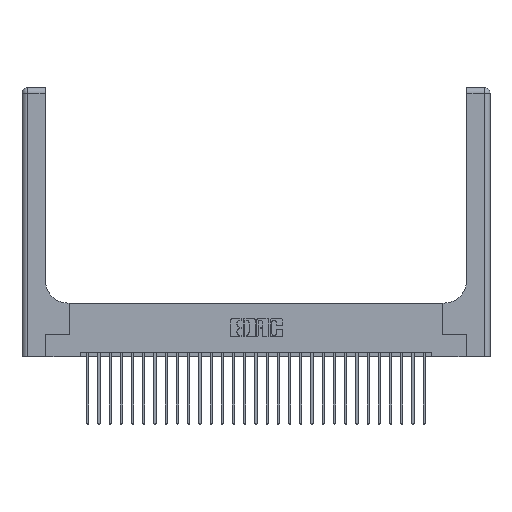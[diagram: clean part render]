
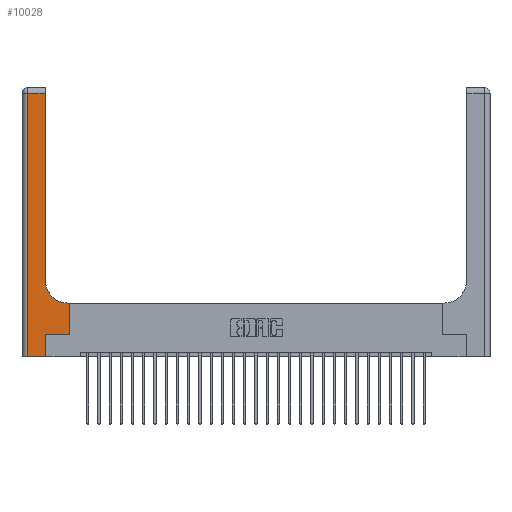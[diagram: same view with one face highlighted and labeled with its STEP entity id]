
A CAD part, top view. The second image highlights one B-rep face of the part: STEP entity #10028.
In plain terms, the highlighted planar face has unit normal (0, 0, 1).
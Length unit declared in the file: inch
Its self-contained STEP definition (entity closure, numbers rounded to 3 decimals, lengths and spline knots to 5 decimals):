
#576 = VERTEX_POINT ( 'NONE', #19433 ) ;
#1052 = CARTESIAN_POINT ( 'NONE',  ( 0.26, 2.94, 0.37 ) ) ;
#1129 = DIRECTION ( 'NONE',  ( 0., 1., 0. ) ) ;
#1941 = CARTESIAN_POINT ( 'NONE',  ( 0.06, 0., 0.37 ) ) ;
#2480 = LINE ( 'NONE', #8867, #11955 ) ;
#2795 = CARTESIAN_POINT ( 'NONE',  ( 0., 3., 0.37 ) ) ;
#3613 = AXIS2_PLACEMENT_3D ( 'NONE', #14170, #26631, #18584 ) ;
#3953 = CARTESIAN_POINT ( 'NONE',  ( 0.265, 0., 0.37 ) ) ;
#4069 = EDGE_CURVE ( 'NONE', #576, #4674, #22612, .T. ) ;
#4525 = ORIENTED_EDGE ( 'NONE', *, *, #26622, .T. ) ;
#4651 = LINE ( 'NONE', #19474, #24740 ) ;
#4674 = VERTEX_POINT ( 'NONE', #25059 ) ;
#4836 = VECTOR ( 'NONE', #20425, 39.37008 ) ;
#4862 = VECTOR ( 'NONE', #7663, 39.37008 ) ;
#5423 = EDGE_CURVE ( 'NONE', #5926, #25636, #27189, .T. ) ;
#5494 = VERTEX_POINT ( 'NONE', #24278 ) ;
#5569 = CARTESIAN_POINT ( 'NONE',  ( 0.51, 0.6, 0.37 ) ) ;
#5577 = VERTEX_POINT ( 'NONE', #5569 ) ;
#5926 = VERTEX_POINT ( 'NONE', #3953 ) ;
#6008 = CARTESIAN_POINT ( 'NONE',  ( 0.265, 0.25, 0.37 ) ) ;
#6046 = CARTESIAN_POINT ( 'NONE',  ( 0., 0., 0.37 ) ) ;
#6304 = ORIENTED_EDGE ( 'NONE', *, *, #6829, .T. ) ;
#6829 = EDGE_CURVE ( 'NONE', #5577, #7321, #22655, .T. ) ;
#7321 = VERTEX_POINT ( 'NONE', #18971 ) ;
#7663 = DIRECTION ( 'NONE',  ( 0., 1., 0. ) ) ;
#8338 = ORIENTED_EDGE ( 'NONE', *, *, #4069, .T. ) ;
#8867 = CARTESIAN_POINT ( 'NONE',  ( 0.265, 0.25, 0.37 ) ) ;
#9286 = VECTOR ( 'NONE', #18909, 39.37008 ) ;
#10028 = ADVANCED_FACE ( 'NONE', ( #27101 ), #26069, .F. ) ;
#10605 = DIRECTION ( 'NONE',  ( -1., 0., 0. ) ) ;
#10785 = VECTOR ( 'NONE', #14510, 39.37008 ) ;
#10938 = DIRECTION ( 'NONE',  ( 1., 0., 0. ) ) ;
#11430 = AXIS2_PLACEMENT_3D ( 'NONE', #2795, #17623, #10605 ) ;
#11649 = EDGE_CURVE ( 'NONE', #5494, #22107, #26661, .T. ) ;
#11955 = VECTOR ( 'NONE', #10938, 39.37008 ) ;
#12024 = EDGE_CURVE ( 'NONE', #7321, #19987, #20126, .T. ) ;
#12362 = VECTOR ( 'NONE', #1129, 39.37008 ) ;
#12437 = ORIENTED_EDGE ( 'NONE', *, *, #18707, .T. ) ;
#14166 = CARTESIAN_POINT ( 'NONE',  ( 0.528, 0.25, 0.37 ) ) ;
#14170 = CARTESIAN_POINT ( 'NONE',  ( 0.51, 0.85, 0.37 ) ) ;
#14466 = CARTESIAN_POINT ( 'NONE',  ( 0.265, 0., 0.37 ) ) ;
#14510 = DIRECTION ( 'NONE',  ( 1., 0., 0. ) ) ;
#15529 = VECTOR ( 'NONE', #18470, 39.37008 ) ;
#16087 = ORIENTED_EDGE ( 'NONE', *, *, #12024, .T. ) ;
#16978 = CARTESIAN_POINT ( 'NONE',  ( 0., 2.94, 0.37 ) ) ;
#17529 = DIRECTION ( 'NONE',  ( -1., 0., 0. ) ) ;
#17623 = DIRECTION ( 'NONE',  ( 0., 0., -1. ) ) ;
#17981 = EDGE_LOOP ( 'NONE', ( #16087, #24592, #23447, #12437, #18421, #4525, #8338, #25033, #6304 ) ) ;
#18421 = ORIENTED_EDGE ( 'NONE', *, *, #5423, .T. ) ;
#18470 = DIRECTION ( 'NONE',  ( 0., 1., 0. ) ) ;
#18584 = DIRECTION ( 'NONE',  ( 1., 0., 0. ) ) ;
#18707 = EDGE_CURVE ( 'NONE', #22107, #5926, #25036, .T. ) ;
#18774 = LINE ( 'NONE', #16978, #9286 ) ;
#18909 = DIRECTION ( 'NONE',  ( -1., 0., 0. ) ) ;
#18971 = CARTESIAN_POINT ( 'NONE',  ( 0.26, 0.85, 0.37 ) ) ;
#19433 = CARTESIAN_POINT ( 'NONE',  ( 0.528, 0.25, 0.37 ) ) ;
#19474 = CARTESIAN_POINT ( 'NONE',  ( 0.26, 0.6, 0.37 ) ) ;
#19987 = VERTEX_POINT ( 'NONE', #1052 ) ;
#20126 = LINE ( 'NONE', #26222, #12362 ) ;
#20425 = DIRECTION ( 'NONE',  ( 0., -1., 0. ) ) ;
#20824 = CARTESIAN_POINT ( 'NONE',  ( 0.06, 3., 0.37 ) ) ;
#22107 = VERTEX_POINT ( 'NONE', #1941 ) ;
#22612 = LINE ( 'NONE', #14166, #4862 ) ;
#22655 = CIRCLE ( 'NONE', #3613, 0.25 ) ;
#23447 = ORIENTED_EDGE ( 'NONE', *, *, #11649, .T. ) ;
#24278 = CARTESIAN_POINT ( 'NONE',  ( 0.06, 2.94, 0.37 ) ) ;
#24592 = ORIENTED_EDGE ( 'NONE', *, *, #25760, .T. ) ;
#24740 = VECTOR ( 'NONE', #17529, 39.37008 ) ;
#25033 = ORIENTED_EDGE ( 'NONE', *, *, #25413, .T. ) ;
#25036 = LINE ( 'NONE', #6046, #10785 ) ;
#25059 = CARTESIAN_POINT ( 'NONE',  ( 0.528, 0.6, 0.37 ) ) ;
#25413 = EDGE_CURVE ( 'NONE', #4674, #5577, #4651, .T. ) ;
#25636 = VERTEX_POINT ( 'NONE', #6008 ) ;
#25760 = EDGE_CURVE ( 'NONE', #19987, #5494, #18774, .T. ) ;
#26069 = PLANE ( 'NONE',  #11430 ) ;
#26222 = CARTESIAN_POINT ( 'NONE',  ( 0.26, 3., 0.37 ) ) ;
#26622 = EDGE_CURVE ( 'NONE', #25636, #576, #2480, .T. ) ;
#26631 = DIRECTION ( 'NONE',  ( 0., 0., -1. ) ) ;
#26661 = LINE ( 'NONE', #20824, #4836 ) ;
#27101 = FACE_OUTER_BOUND ( 'NONE', #17981, .T. ) ;
#27189 = LINE ( 'NONE', #14466, #15529 ) ;
